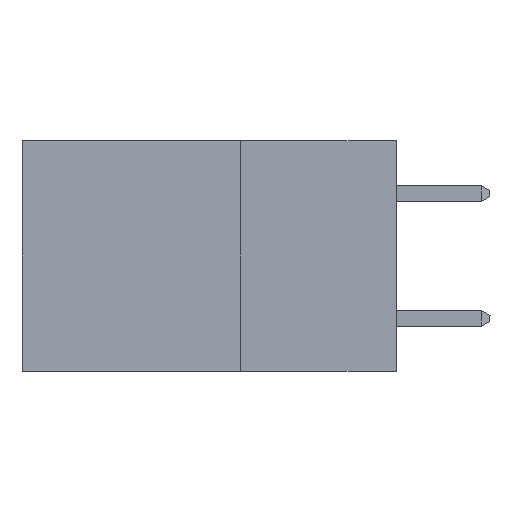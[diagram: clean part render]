
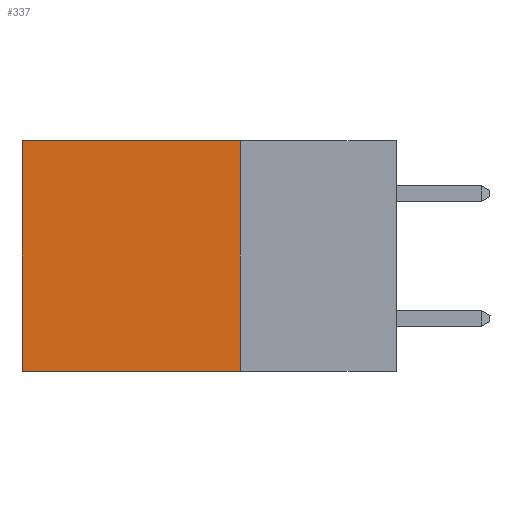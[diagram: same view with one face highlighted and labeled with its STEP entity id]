
A CAD part, left-side view. The second image highlights one B-rep face of the part: STEP entity #337.
In plain terms, the highlighted planar face has unit normal (-1, 0, 0).
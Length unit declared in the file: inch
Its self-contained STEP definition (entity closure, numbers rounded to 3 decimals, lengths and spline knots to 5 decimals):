
#337 = ADVANCED_FACE ( 'NONE', ( #10921 ), #8864, .F. ) ;
#428 = EDGE_CURVE ( 'NONE', #8581, #2822, #3074, .T. ) ;
#758 = LINE ( 'NONE', #6985, #2699 ) ;
#839 = AXIS2_PLACEMENT_3D ( 'NONE', #5628, #6655, #6716 ) ;
#1142 = CARTESIAN_POINT ( 'NONE',  ( 0.298, 0.6, 0. ) ) ;
#1626 = VECTOR ( 'NONE', #3321, 39.37008 ) ;
#2058 = EDGE_CURVE ( 'NONE', #8581, #10927, #758, .T. ) ;
#2699 = VECTOR ( 'NONE', #9225, 39.37008 ) ;
#2772 = DIRECTION ( 'NONE',  ( 0., 1., 0. ) ) ;
#2796 = ORIENTED_EDGE ( 'NONE', *, *, #428, .T. ) ;
#2822 = VERTEX_POINT ( 'NONE', #11305 ) ;
#3074 = LINE ( 'NONE', #5275, #14397 ) ;
#3321 = DIRECTION ( 'NONE',  ( 0., 0., -1. ) ) ;
#3529 = EDGE_CURVE ( 'NONE', #2822, #11146, #7480, .T. ) ;
#5275 = CARTESIAN_POINT ( 'NONE',  ( 0.298, 0.25, 0. ) ) ;
#5392 = CARTESIAN_POINT ( 'NONE',  ( 0.298, 0.25, 0. ) ) ;
#5628 = CARTESIAN_POINT ( 'NONE',  ( 0.298, 0.25, 0. ) ) ;
#6372 = ORIENTED_EDGE ( 'NONE', *, *, #7518, .F. ) ;
#6430 = VECTOR ( 'NONE', #2772, 39.37008 ) ;
#6655 = DIRECTION ( 'NONE',  ( 1., 0., 0. ) ) ;
#6716 = DIRECTION ( 'NONE',  ( 0., 0., -1. ) ) ;
#6959 = CARTESIAN_POINT ( 'NONE',  ( 0.298, 0.25, -0.37 ) ) ;
#6985 = CARTESIAN_POINT ( 'NONE',  ( 0.298, 0.25, 0. ) ) ;
#7480 = LINE ( 'NONE', #1142, #1626 ) ;
#7488 = LINE ( 'NONE', #10450, #6430 ) ;
#7518 = EDGE_CURVE ( 'NONE', #10927, #11146, #7488, .T. ) ;
#7924 = EDGE_LOOP ( 'NONE', ( #8661, #6372, #14088, #2796 ) ) ;
#8581 = VERTEX_POINT ( 'NONE', #5392 ) ;
#8661 = ORIENTED_EDGE ( 'NONE', *, *, #3529, .T. ) ;
#8864 = PLANE ( 'NONE',  #839 ) ;
#9225 = DIRECTION ( 'NONE',  ( 0., 0., -1. ) ) ;
#10450 = CARTESIAN_POINT ( 'NONE',  ( 0.298, 0.25, -0.37 ) ) ;
#10921 = FACE_OUTER_BOUND ( 'NONE', #7924, .T. ) ;
#10927 = VERTEX_POINT ( 'NONE', #6959 ) ;
#11146 = VERTEX_POINT ( 'NONE', #12724 ) ;
#11305 = CARTESIAN_POINT ( 'NONE',  ( 0.298, 0.6, 0. ) ) ;
#12724 = CARTESIAN_POINT ( 'NONE',  ( 0.298, 0.6, -0.37 ) ) ;
#13178 = DIRECTION ( 'NONE',  ( 0., 1., 0. ) ) ;
#14088 = ORIENTED_EDGE ( 'NONE', *, *, #2058, .F. ) ;
#14397 = VECTOR ( 'NONE', #13178, 39.37008 ) ;
